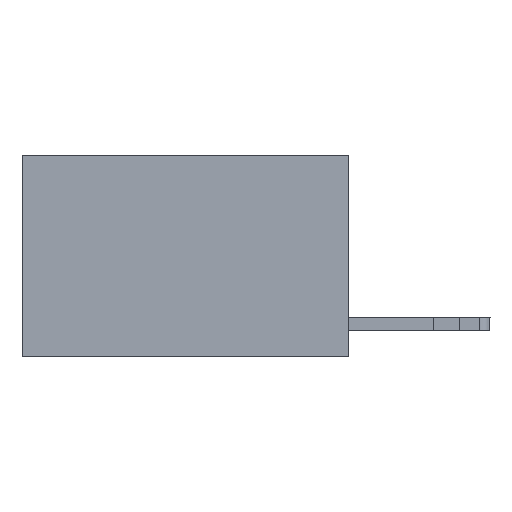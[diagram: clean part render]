
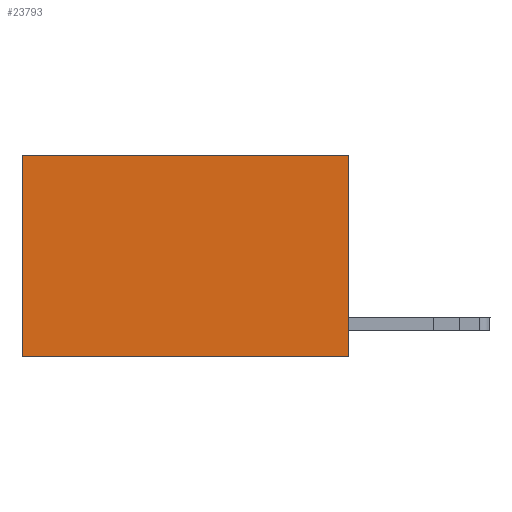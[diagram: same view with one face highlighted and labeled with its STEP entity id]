
A CAD part, left-side view. The second image highlights one B-rep face of the part: STEP entity #23793.
In plain terms, the highlighted planar face has unit normal (-1, 0, 0).
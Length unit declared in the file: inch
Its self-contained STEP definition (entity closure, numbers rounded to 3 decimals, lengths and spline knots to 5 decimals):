
#617 = CARTESIAN_POINT ( 'NONE',  ( 0.2625, 0.6, 0. ) ) ;
#628 = VERTEX_POINT ( 'NONE', #16133 ) ;
#1089 = DIRECTION ( 'NONE',  ( 0., 1., 0. ) ) ;
#1166 = DIRECTION ( 'NONE',  ( 0., 0., -1. ) ) ;
#1283 = LINE ( 'NONE', #25683, #21962 ) ;
#1327 = DIRECTION ( 'NONE',  ( 0., 0., -1. ) ) ;
#1870 = DIRECTION ( 'NONE',  ( 0., 0., -1. ) ) ;
#4188 = VECTOR ( 'NONE', #6679, 39.37008 ) ;
#4642 = EDGE_CURVE ( 'NONE', #24898, #628, #25239, .T. ) ;
#4708 = ORIENTED_EDGE ( 'NONE', *, *, #26663, .F. ) ;
#6146 = VECTOR ( 'NONE', #1870, 39.37008 ) ;
#6679 = DIRECTION ( 'NONE',  ( 0., 1., 0. ) ) ;
#7476 = CARTESIAN_POINT ( 'NONE',  ( 0.2625, 0., 0. ) ) ;
#11386 = ORIENTED_EDGE ( 'NONE', *, *, #4642, .T. ) ;
#11461 = CARTESIAN_POINT ( 'NONE',  ( 0.2625, 0.6, 0. ) ) ;
#13372 = VERTEX_POINT ( 'NONE', #25682 ) ;
#13479 = ORIENTED_EDGE ( 'NONE', *, *, #22128, .F. ) ;
#13725 = DIRECTION ( 'NONE',  ( 1., 0., 0. ) ) ;
#14315 = VECTOR ( 'NONE', #1166, 39.37008 ) ;
#14512 = AXIS2_PLACEMENT_3D ( 'NONE', #7476, #13725, #1327 ) ;
#15488 = FACE_OUTER_BOUND ( 'NONE', #25757, .T. ) ;
#16133 = CARTESIAN_POINT ( 'NONE',  ( 0.2625, 0.6, -0.37 ) ) ;
#16529 = LINE ( 'NONE', #20366, #6146 ) ;
#16997 = CARTESIAN_POINT ( 'NONE',  ( 0.2625, 0., -0.37 ) ) ;
#19845 = CARTESIAN_POINT ( 'NONE',  ( 0.2625, 0., 0. ) ) ;
#20366 = CARTESIAN_POINT ( 'NONE',  ( 0.2625, 0., 0. ) ) ;
#21962 = VECTOR ( 'NONE', #1089, 39.37008 ) ;
#22128 = EDGE_CURVE ( 'NONE', #13372, #628, #25468, .T. ) ;
#22442 = VERTEX_POINT ( 'NONE', #19845 ) ;
#23096 = EDGE_CURVE ( 'NONE', #22442, #24898, #1283, .T. ) ;
#23793 = ADVANCED_FACE ( 'NONE', ( #15488 ), #26000, .F. ) ;
#24813 = ORIENTED_EDGE ( 'NONE', *, *, #23096, .T. ) ;
#24898 = VERTEX_POINT ( 'NONE', #617 ) ;
#25239 = LINE ( 'NONE', #11461, #14315 ) ;
#25468 = LINE ( 'NONE', #16997, #4188 ) ;
#25682 = CARTESIAN_POINT ( 'NONE',  ( 0.2625, 0., -0.37 ) ) ;
#25683 = CARTESIAN_POINT ( 'NONE',  ( 0.2625, 0., 0. ) ) ;
#25757 = EDGE_LOOP ( 'NONE', ( #11386, #13479, #4708, #24813 ) ) ;
#26000 = PLANE ( 'NONE',  #14512 ) ;
#26663 = EDGE_CURVE ( 'NONE', #22442, #13372, #16529, .T. ) ;
